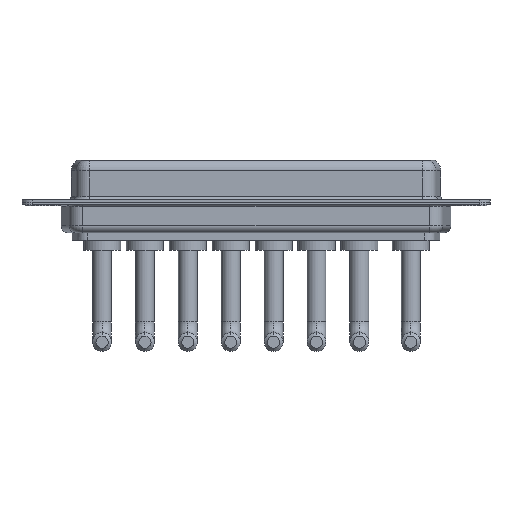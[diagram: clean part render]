
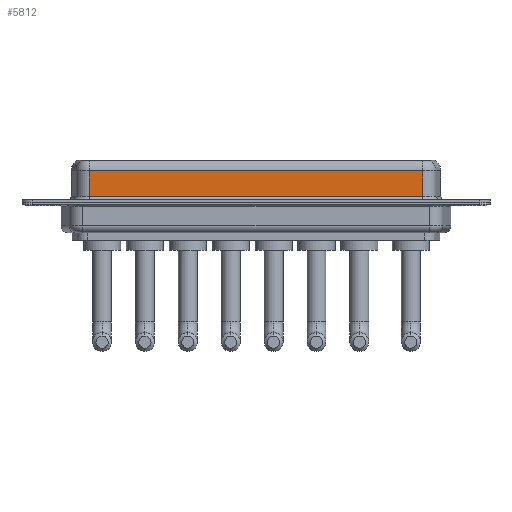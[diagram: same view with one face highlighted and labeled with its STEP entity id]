
A CAD part, front view. The second image highlights one B-rep face of the part: STEP entity #5812.
In plain terms, the highlighted planar face has unit normal (0, -1, 0).
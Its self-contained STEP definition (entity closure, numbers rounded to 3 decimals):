
#408 = VERTEX_POINT ( 'NONE', #8433 ) ;
#697 = CARTESIAN_POINT ( 'NONE',  ( 56.462, -3.95, 4.65 ) ) ;
#1009 = CARTESIAN_POINT ( 'NONE',  ( 56.462, -3.95, 6.4 ) ) ;
#1306 = LINE ( 'NONE', #697, #5863 ) ;
#1836 = DIRECTION ( 'NONE',  ( 0., 1., 0. ) ) ;
#2210 = DIRECTION ( 'NONE',  ( 1., 0., 0. ) ) ;
#2966 = CARTESIAN_POINT ( 'NONE',  ( 7.038, -3.95, 6.4 ) ) ;
#3138 = CARTESIAN_POINT ( 'NONE',  ( 56.462, -3.95, 0.9 ) ) ;
#4185 = LINE ( 'NONE', #3138, #8971 ) ;
#4756 = DIRECTION ( 'NONE',  ( 0., 0., -1. ) ) ;
#4783 = DIRECTION ( 'NONE',  ( 0., 0., -1. ) ) ;
#5362 = FACE_OUTER_BOUND ( 'NONE', #10797, .T. ) ;
#5584 = DIRECTION ( 'NONE',  ( 0., 0., 1. ) ) ;
#5752 = ORIENTED_EDGE ( 'NONE', *, *, #9845, .F. ) ;
#5812 = ADVANCED_FACE ( 'NONE', ( #5362 ), #8982, .F. ) ;
#5863 = VECTOR ( 'NONE', #5972, 1000. ) ;
#5938 = ORIENTED_EDGE ( 'NONE', *, *, #10943, .T. ) ;
#5972 = DIRECTION ( 'NONE',  ( -1., 0., 0. ) ) ;
#6222 = EDGE_CURVE ( 'NONE', #10848, #408, #7391, .T. ) ;
#7113 = ORIENTED_EDGE ( 'NONE', *, *, #6222, .T. ) ;
#7391 = LINE ( 'NONE', #2966, #8354 ) ;
#7528 = CARTESIAN_POINT ( 'NONE',  ( 56.462, -3.95, 6.4 ) ) ;
#7590 = EDGE_CURVE ( 'NONE', #408, #10164, #4185, .T. ) ;
#7794 = ORIENTED_EDGE ( 'NONE', *, *, #7590, .T. ) ;
#8215 = CARTESIAN_POINT ( 'NONE',  ( 56.462, -3.95, 4.65 ) ) ;
#8354 = VECTOR ( 'NONE', #4756, 1000. ) ;
#8389 = LINE ( 'NONE', #7528, #11421 ) ;
#8433 = CARTESIAN_POINT ( 'NONE',  ( 7.038, -3.95, 0.9 ) ) ;
#8535 = VERTEX_POINT ( 'NONE', #8215 ) ;
#8610 = CARTESIAN_POINT ( 'NONE',  ( 7.038, -3.95, 4.65 ) ) ;
#8971 = VECTOR ( 'NONE', #2210, 1000. ) ;
#8982 = PLANE ( 'NONE',  #11453 ) ;
#9845 = EDGE_CURVE ( 'NONE', #8535, #10164, #8389, .T. ) ;
#10164 = VERTEX_POINT ( 'NONE', #10588 ) ;
#10588 = CARTESIAN_POINT ( 'NONE',  ( 56.462, -3.95, 0.9 ) ) ;
#10797 = EDGE_LOOP ( 'NONE', ( #5752, #5938, #7113, #7794 ) ) ;
#10848 = VERTEX_POINT ( 'NONE', #8610 ) ;
#10943 = EDGE_CURVE ( 'NONE', #8535, #10848, #1306, .T. ) ;
#11421 = VECTOR ( 'NONE', #4783, 1000. ) ;
#11453 = AXIS2_PLACEMENT_3D ( 'NONE', #1009, #1836, #5584 ) ;
